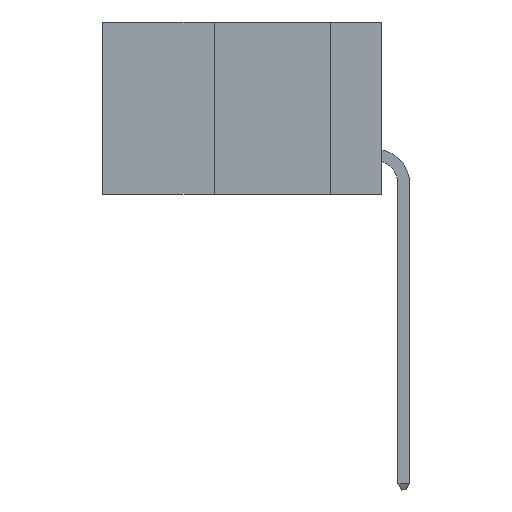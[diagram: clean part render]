
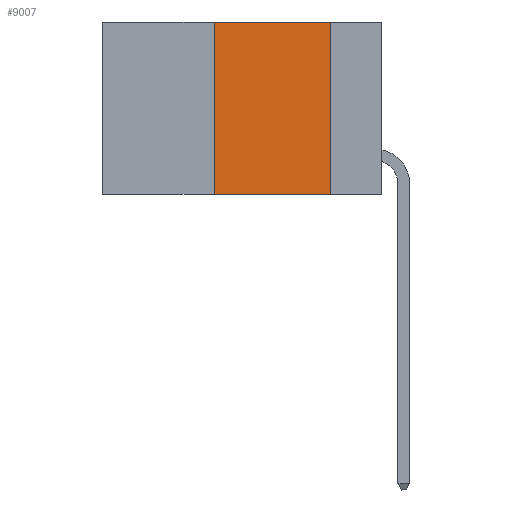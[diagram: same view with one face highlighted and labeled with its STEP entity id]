
A CAD part, left-side view. The second image highlights one B-rep face of the part: STEP entity #9007.
In plain terms, the highlighted planar face has unit normal (-1, 0, 0).
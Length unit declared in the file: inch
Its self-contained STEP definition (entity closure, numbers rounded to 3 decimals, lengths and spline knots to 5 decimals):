
#317 = CARTESIAN_POINT ( 'NONE',  ( 0., 0.11, 0. ) ) ;
#557 = DIRECTION ( 'NONE',  ( 1., 0., 0. ) ) ;
#829 = VECTOR ( 'NONE', #10053, 39.37008 ) ;
#1758 = CARTESIAN_POINT ( 'NONE',  ( 0., 0.11, -0.37 ) ) ;
#1780 = VECTOR ( 'NONE', #9699, 39.37008 ) ;
#1937 = VERTEX_POINT ( 'NONE', #1980 ) ;
#1980 = CARTESIAN_POINT ( 'NONE',  ( 0., 0.36, 0. ) ) ;
#2182 = VERTEX_POINT ( 'NONE', #1758 ) ;
#2412 = DIRECTION ( 'NONE',  ( 0., -1., 0. ) ) ;
#2431 = VERTEX_POINT ( 'NONE', #317 ) ;
#2679 = FACE_OUTER_BOUND ( 'NONE', #2899, .T. ) ;
#2899 = EDGE_LOOP ( 'NONE', ( #9240, #10748, #9720, #6883 ) ) ;
#3117 = CARTESIAN_POINT ( 'NONE',  ( 0., 0.6, 0. ) ) ;
#3394 = EDGE_CURVE ( 'NONE', #2431, #2182, #9957, .T. ) ;
#3862 = EDGE_CURVE ( 'NONE', #1937, #2431, #10693, .T. ) ;
#5105 = LINE ( 'NONE', #7406, #6793 ) ;
#5497 = CARTESIAN_POINT ( 'NONE',  ( 0., 0.36, 0. ) ) ;
#5875 = EDGE_CURVE ( 'NONE', #10454, #2182, #5105, .T. ) ;
#6333 = LINE ( 'NONE', #5497, #1780 ) ;
#6359 = PLANE ( 'NONE',  #6738 ) ;
#6397 = DIRECTION ( 'NONE',  ( 0., 0., -1. ) ) ;
#6547 = CARTESIAN_POINT ( 'NONE',  ( 0., 0.11, 0. ) ) ;
#6738 = AXIS2_PLACEMENT_3D ( 'NONE', #3117, #557, #6397 ) ;
#6751 = CARTESIAN_POINT ( 'NONE',  ( 0., 0.6, 0. ) ) ;
#6793 = VECTOR ( 'NONE', #2412, 39.37008 ) ;
#6883 = ORIENTED_EDGE ( 'NONE', *, *, #5875, .T. ) ;
#7174 = CARTESIAN_POINT ( 'NONE',  ( 0., 0.36, -0.37 ) ) ;
#7406 = CARTESIAN_POINT ( 'NONE',  ( 0., 0.6, -0.37 ) ) ;
#7755 = VECTOR ( 'NONE', #9925, 39.37008 ) ;
#8056 = EDGE_CURVE ( 'NONE', #10454, #1937, #6333, .T. ) ;
#9007 = ADVANCED_FACE ( 'NONE', ( #2679 ), #6359, .F. ) ;
#9240 = ORIENTED_EDGE ( 'NONE', *, *, #3394, .F. ) ;
#9699 = DIRECTION ( 'NONE',  ( 0., 0., 1. ) ) ;
#9720 = ORIENTED_EDGE ( 'NONE', *, *, #8056, .F. ) ;
#9925 = DIRECTION ( 'NONE',  ( 0., 0., -1. ) ) ;
#9957 = LINE ( 'NONE', #6547, #7755 ) ;
#10053 = DIRECTION ( 'NONE',  ( 0., -1., 0. ) ) ;
#10454 = VERTEX_POINT ( 'NONE', #7174 ) ;
#10693 = LINE ( 'NONE', #6751, #829 ) ;
#10748 = ORIENTED_EDGE ( 'NONE', *, *, #3862, .F. ) ;
